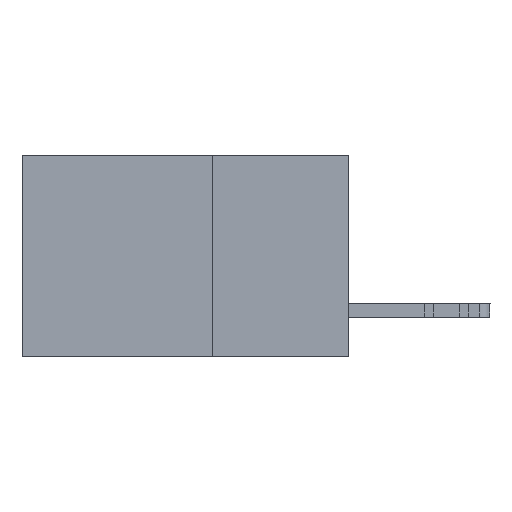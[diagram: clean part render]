
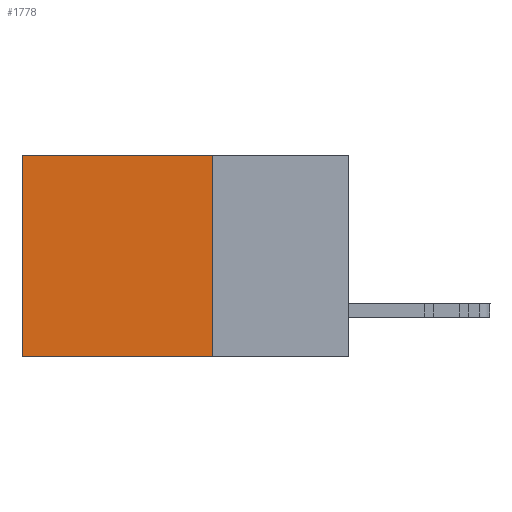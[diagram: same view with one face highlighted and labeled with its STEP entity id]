
A CAD part, left-side view. The second image highlights one B-rep face of the part: STEP entity #1778.
In plain terms, the highlighted planar face has unit normal (-1, 0, 0).
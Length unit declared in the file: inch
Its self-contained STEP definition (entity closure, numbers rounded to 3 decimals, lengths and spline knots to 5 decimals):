
#180 = VERTEX_POINT ( 'NONE', #14009 ) ;
#636 = EDGE_CURVE ( 'NONE', #7215, #2205, #15535, .T. ) ;
#1653 = VECTOR ( 'NONE', #16604, 39.37008 ) ;
#1778 = ADVANCED_FACE ( 'NONE', ( #22485 ), #21614, .F. ) ;
#1932 = DIRECTION ( 'NONE',  ( 0., 0., -1. ) ) ;
#1973 = DIRECTION ( 'NONE',  ( 1., 0., 0. ) ) ;
#2205 = VERTEX_POINT ( 'NONE', #11145 ) ;
#2797 = LINE ( 'NONE', #11177, #1653 ) ;
#3395 = DIRECTION ( 'NONE',  ( 0., 0., -1. ) ) ;
#4103 = DIRECTION ( 'NONE',  ( 0., 1., 0. ) ) ;
#7215 = VERTEX_POINT ( 'NONE', #8272 ) ;
#7969 = LINE ( 'NONE', #15227, #17711 ) ;
#8272 = CARTESIAN_POINT ( 'NONE',  ( 0.2615, 0.25, 0. ) ) ;
#8314 = VECTOR ( 'NONE', #11540, 39.37008 ) ;
#8902 = CARTESIAN_POINT ( 'NONE',  ( 0.2615, 0.25, -0.37 ) ) ;
#10335 = AXIS2_PLACEMENT_3D ( 'NONE', #8902, #1973, #1932 ) ;
#11145 = CARTESIAN_POINT ( 'NONE',  ( 0.2615, 0.25, -0.37 ) ) ;
#11177 = CARTESIAN_POINT ( 'NONE',  ( 0.2615, 0.25, 0. ) ) ;
#11420 = EDGE_CURVE ( 'NONE', #180, #18560, #13188, .T. ) ;
#11540 = DIRECTION ( 'NONE',  ( 0., 0., -1. ) ) ;
#13188 = LINE ( 'NONE', #18801, #8314 ) ;
#13512 = CARTESIAN_POINT ( 'NONE',  ( 0.2615, 0.25, -0.37 ) ) ;
#14009 = CARTESIAN_POINT ( 'NONE',  ( 0.2615, 0.6, 0. ) ) ;
#15227 = CARTESIAN_POINT ( 'NONE',  ( 0.2615, 0.25, -0.37 ) ) ;
#15535 = LINE ( 'NONE', #13512, #19221 ) ;
#15820 = EDGE_CURVE ( 'NONE', #7215, #180, #2797, .T. ) ;
#15881 = ORIENTED_EDGE ( 'NONE', *, *, #636, .F. ) ;
#15933 = ORIENTED_EDGE ( 'NONE', *, *, #19117, .F. ) ;
#16175 = ORIENTED_EDGE ( 'NONE', *, *, #15820, .T. ) ;
#16604 = DIRECTION ( 'NONE',  ( 0., 1., 0. ) ) ;
#17320 = CARTESIAN_POINT ( 'NONE',  ( 0.2615, 0.6, -0.37 ) ) ;
#17711 = VECTOR ( 'NONE', #4103, 39.37008 ) ;
#18560 = VERTEX_POINT ( 'NONE', #17320 ) ;
#18801 = CARTESIAN_POINT ( 'NONE',  ( 0.2615, 0.6, -0.37 ) ) ;
#19117 = EDGE_CURVE ( 'NONE', #2205, #18560, #7969, .T. ) ;
#19221 = VECTOR ( 'NONE', #3395, 39.37008 ) ;
#21614 = PLANE ( 'NONE',  #10335 ) ;
#21843 = EDGE_LOOP ( 'NONE', ( #22569, #15933, #15881, #16175 ) ) ;
#22485 = FACE_OUTER_BOUND ( 'NONE', #21843, .T. ) ;
#22569 = ORIENTED_EDGE ( 'NONE', *, *, #11420, .T. ) ;
